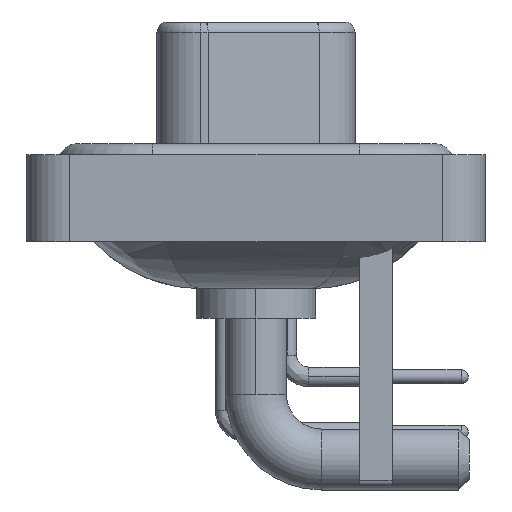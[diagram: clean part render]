
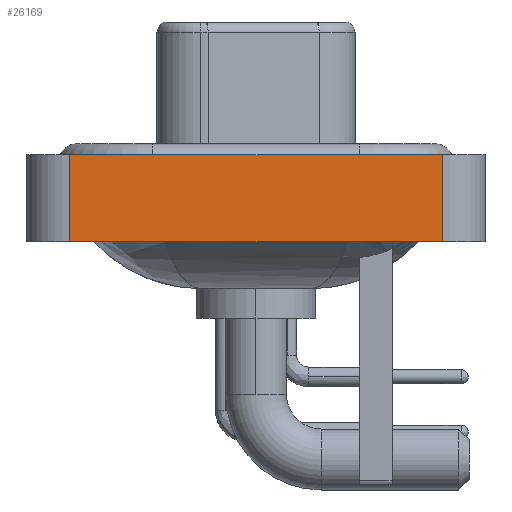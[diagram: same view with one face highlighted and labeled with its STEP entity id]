
A CAD part, left-side view. The second image highlights one B-rep face of the part: STEP entity #26169.
In plain terms, the highlighted planar face has unit normal (-1, 0, 0).
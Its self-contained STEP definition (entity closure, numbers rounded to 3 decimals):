
#556 = DIRECTION ( 'NONE',  ( 0., 0., 1. ) ) ;
#1613 = ORIENTED_EDGE ( 'NONE', *, *, #11403, .T. ) ;
#2673 = VECTOR ( 'NONE', #24438, 1000. ) ;
#2708 = CARTESIAN_POINT ( 'NONE',  ( -7.35, -8.55, -3.6 ) ) ;
#4070 = VECTOR ( 'NONE', #17296, 1000. ) ;
#4386 = VERTEX_POINT ( 'NONE', #17770 ) ;
#5605 = EDGE_CURVE ( 'NONE', #4386, #16159, #13193, .T. ) ;
#7087 = DIRECTION ( 'NONE',  ( 0., 0., 1. ) ) ;
#9205 = VECTOR ( 'NONE', #12967, 1000. ) ;
#10465 = EDGE_CURVE ( 'NONE', #16060, #16159, #19239, .T. ) ;
#10868 = FACE_OUTER_BOUND ( 'NONE', #25852, .T. ) ;
#11403 = EDGE_CURVE ( 'NONE', #26185, #4386, #19606, .T. ) ;
#12794 = VECTOR ( 'NONE', #7087, 1000. ) ;
#12967 = DIRECTION ( 'NONE',  ( 0., -1., 0. ) ) ;
#13062 = CARTESIAN_POINT ( 'NONE',  ( -7.35, -8.55, -3.6 ) ) ;
#13193 = LINE ( 'NONE', #13062, #12794 ) ;
#13316 = AXIS2_PLACEMENT_3D ( 'NONE', #2708, #19165, #556 ) ;
#16060 = VERTEX_POINT ( 'NONE', #19204 ) ;
#16159 = VERTEX_POINT ( 'NONE', #17274 ) ;
#16436 = ORIENTED_EDGE ( 'NONE', *, *, #20841, .F. ) ;
#17274 = CARTESIAN_POINT ( 'NONE',  ( -7.35, -8.55, 0.4 ) ) ;
#17296 = DIRECTION ( 'NONE',  ( 0., -1., 0. ) ) ;
#17435 = CARTESIAN_POINT ( 'NONE',  ( -7.35, -8.55, -3.6 ) ) ;
#17770 = CARTESIAN_POINT ( 'NONE',  ( -7.35, -8.55, -3.6 ) ) ;
#18570 = CARTESIAN_POINT ( 'NONE',  ( -7.35, 8.55, -3.6 ) ) ;
#19165 = DIRECTION ( 'NONE',  ( -1., 0., 0. ) ) ;
#19204 = CARTESIAN_POINT ( 'NONE',  ( -7.35, 8.55, 0.4 ) ) ;
#19239 = LINE ( 'NONE', #25762, #9205 ) ;
#19606 = LINE ( 'NONE', #17435, #4070 ) ;
#20841 = EDGE_CURVE ( 'NONE', #26185, #16060, #24702, .T. ) ;
#23135 = PLANE ( 'NONE',  #13316 ) ;
#24141 = ORIENTED_EDGE ( 'NONE', *, *, #5605, .T. ) ;
#24438 = DIRECTION ( 'NONE',  ( 0., 0., 1. ) ) ;
#24702 = LINE ( 'NONE', #18570, #2673 ) ;
#25415 = CARTESIAN_POINT ( 'NONE',  ( -7.35, 8.55, -3.6 ) ) ;
#25762 = CARTESIAN_POINT ( 'NONE',  ( -7.35, -8.55, 0.4 ) ) ;
#25852 = EDGE_LOOP ( 'NONE', ( #24141, #26145, #16436, #1613 ) ) ;
#26145 = ORIENTED_EDGE ( 'NONE', *, *, #10465, .F. ) ;
#26169 = ADVANCED_FACE ( 'NONE', ( #10868 ), #23135, .T. ) ;
#26185 = VERTEX_POINT ( 'NONE', #25415 ) ;
